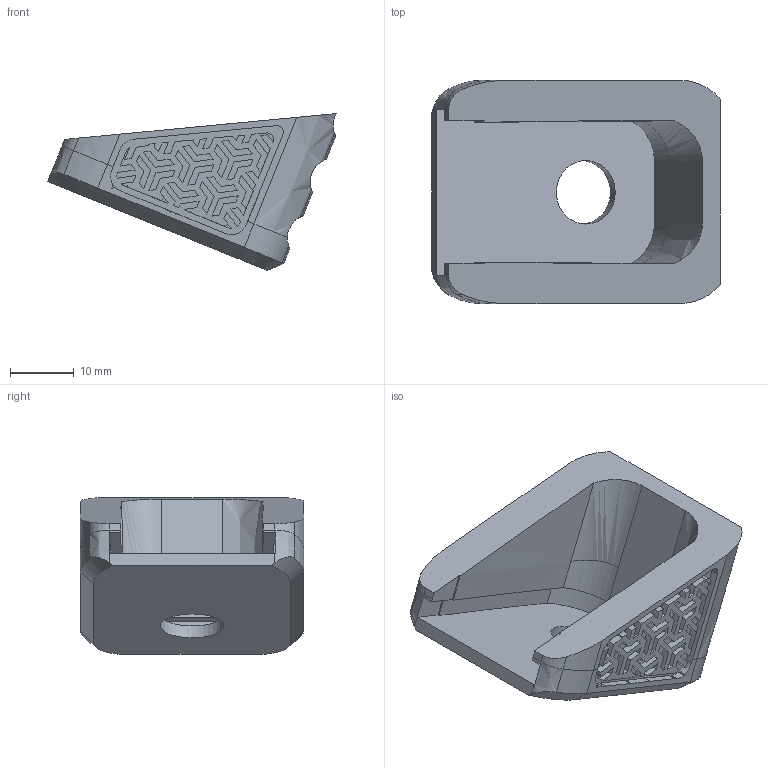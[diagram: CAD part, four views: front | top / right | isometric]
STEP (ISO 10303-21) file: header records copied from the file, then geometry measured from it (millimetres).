
FILE_DESCRIPTION(/* description */ (''),/* implementation_level */ '2;1');
FILE_NAME(/* name */ 'Base Plate.step',/* time_stamp */ '2022-05-12T10:51:25-06:00',/* author */ (''),/* organization */ (''),/* preprocessor_version */ 'ST-DEVELOPER v18.1',/* originating_system */ 'Autodesk Translation Framework v10.10.0.1391',/* authorisation */ '');
FILE_SCHEMA (('AUTOMOTIVE_DESIGN { 1 0 10303 214 3 1 1 }'));
Length unit declared in the file: millimetre
Products named in the file (1): end plate
Bounding box: 45.4 x 35.13 x 24.67 mm (x, y, z)
Volume: 10442.8 mm3; surface area: 7445.2 mm2
Topology: 1 solids, 1 shells, 527 faces, 1454 edges, 961 vertices
Faces by surface type: plane 451, bspline 44, cylinder 32
Full cylindrical faces by diameter (mm): 10 x1
Entity records: 23983 total; most frequent: CARTESIAN_POINT 10914, ORIENTED_EDGE 2908, DIRECTION 2309, EDGE_CURVE 1454, LINE 1233, VECTOR 1233, VERTEX_POINT 961, EDGE_LOOP 561
